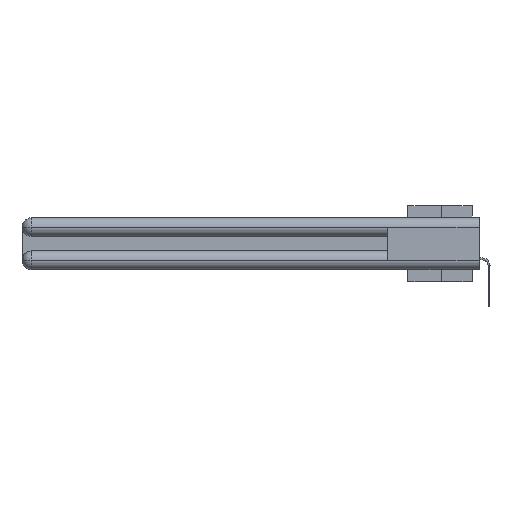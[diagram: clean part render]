
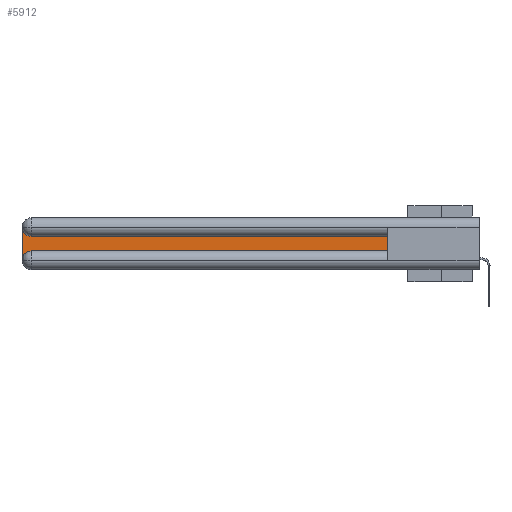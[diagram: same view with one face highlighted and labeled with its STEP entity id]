
A CAD part, left-side view. The second image highlights one B-rep face of the part: STEP entity #5912.
In plain terms, the highlighted planar face has unit normal (-1, 0, 0).
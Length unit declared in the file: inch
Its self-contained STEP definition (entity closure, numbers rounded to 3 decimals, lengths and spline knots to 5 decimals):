
#615 = CARTESIAN_POINT ( 'NONE',  ( 0.075, 0.6, -0.2175 ) ) ;
#784 = CARTESIAN_POINT ( 'NONE',  ( 0.075, 0.6, -0.1225 ) ) ;
#956 = DIRECTION ( 'NONE',  ( 1., 0., 0. ) ) ;
#1449 = CARTESIAN_POINT ( 'NONE',  ( 0.075, 3., -0.1225 ) ) ;
#1852 = ORIENTED_EDGE ( 'NONE', *, *, #7836, .T. ) ;
#2222 = DIRECTION ( 'NONE',  ( 0., 0., -1. ) ) ;
#2273 = EDGE_CURVE ( 'NONE', #6362, #12869, #2788, .T. ) ;
#2788 = LINE ( 'NONE', #10233, #27719 ) ;
#4171 = CARTESIAN_POINT ( 'NONE',  ( 0.075, 2.94, -0.0625 ) ) ;
#4339 = DIRECTION ( 'NONE',  ( 1., 0., 0. ) ) ;
#5912 = ADVANCED_FACE ( 'NONE', ( #26158 ), #13290, .F. ) ;
#6362 = VERTEX_POINT ( 'NONE', #11293 ) ;
#7059 = LINE ( 'NONE', #24300, #19190 ) ;
#7089 = LINE ( 'NONE', #29381, #31276 ) ;
#7391 = EDGE_CURVE ( 'NONE', #25984, #6362, #17122, .T. ) ;
#7774 = AXIS2_PLACEMENT_3D ( 'NONE', #17007, #16689, #21905 ) ;
#7794 = DIRECTION ( 'NONE',  ( 0., -1., 0. ) ) ;
#7836 = EDGE_CURVE ( 'NONE', #12869, #9637, #7059, .T. ) ;
#8043 = ORIENTED_EDGE ( 'NONE', *, *, #19424, .T. ) ;
#8418 = DIRECTION ( 'NONE',  ( 0., 0., -1. ) ) ;
#8430 = VECTOR ( 'NONE', #13844, 39.37008 ) ;
#8627 = EDGE_CURVE ( 'NONE', #10964, #16757, #12493, .T. ) ;
#9637 = VERTEX_POINT ( 'NONE', #784 ) ;
#10233 = CARTESIAN_POINT ( 'NONE',  ( 0.075, 0.6, -0.2175 ) ) ;
#10964 = VERTEX_POINT ( 'NONE', #25983 ) ;
#11293 = CARTESIAN_POINT ( 'NONE',  ( 0.075, 2.94, -0.2175 ) ) ;
#11928 = EDGE_CURVE ( 'NONE', #16757, #25984, #23780, .T. ) ;
#12493 = CIRCLE ( 'NONE', #29119, 0.06 ) ;
#12676 = EDGE_LOOP ( 'NONE', ( #8043, #30890, #13658, #15280, #29915, #1852 ) ) ;
#12869 = VERTEX_POINT ( 'NONE', #615 ) ;
#13290 = PLANE ( 'NONE',  #20217 ) ;
#13658 = ORIENTED_EDGE ( 'NONE', *, *, #11928, .T. ) ;
#13844 = DIRECTION ( 'NONE',  ( 0., 0., -1. ) ) ;
#14557 = DIRECTION ( 'NONE',  ( 0., 1., 0. ) ) ;
#15280 = ORIENTED_EDGE ( 'NONE', *, *, #7391, .T. ) ;
#16689 = DIRECTION ( 'NONE',  ( 1., 0., 0. ) ) ;
#16757 = VERTEX_POINT ( 'NONE', #17109 ) ;
#17007 = CARTESIAN_POINT ( 'NONE',  ( 0.075, 2.94, -0.2775 ) ) ;
#17109 = CARTESIAN_POINT ( 'NONE',  ( 0.075, 3., -0.0625 ) ) ;
#17122 = CIRCLE ( 'NONE', #7774, 0.06 ) ;
#19190 = VECTOR ( 'NONE', #27068, 39.37008 ) ;
#19424 = EDGE_CURVE ( 'NONE', #9637, #10964, #7089, .T. ) ;
#20217 = AXIS2_PLACEMENT_3D ( 'NONE', #1449, #956, #8418 ) ;
#21905 = DIRECTION ( 'NONE',  ( 0., 0., -1. ) ) ;
#23780 = LINE ( 'NONE', #28681, #8430 ) ;
#24300 = CARTESIAN_POINT ( 'NONE',  ( 0.075, 0.6, -0.2175 ) ) ;
#25983 = CARTESIAN_POINT ( 'NONE',  ( 0.075, 2.94, -0.1225 ) ) ;
#25984 = VERTEX_POINT ( 'NONE', #28770 ) ;
#26158 = FACE_OUTER_BOUND ( 'NONE', #12676, .T. ) ;
#27068 = DIRECTION ( 'NONE',  ( 0., 0., 1. ) ) ;
#27719 = VECTOR ( 'NONE', #7794, 39.37008 ) ;
#28681 = CARTESIAN_POINT ( 'NONE',  ( 0.075, 3., -0.2175 ) ) ;
#28770 = CARTESIAN_POINT ( 'NONE',  ( 0.075, 3., -0.2775 ) ) ;
#29119 = AXIS2_PLACEMENT_3D ( 'NONE', #4171, #4339, #2222 ) ;
#29381 = CARTESIAN_POINT ( 'NONE',  ( 0.075, 0.6, -0.1225 ) ) ;
#29915 = ORIENTED_EDGE ( 'NONE', *, *, #2273, .T. ) ;
#30890 = ORIENTED_EDGE ( 'NONE', *, *, #8627, .T. ) ;
#31276 = VECTOR ( 'NONE', #14557, 39.37008 ) ;
